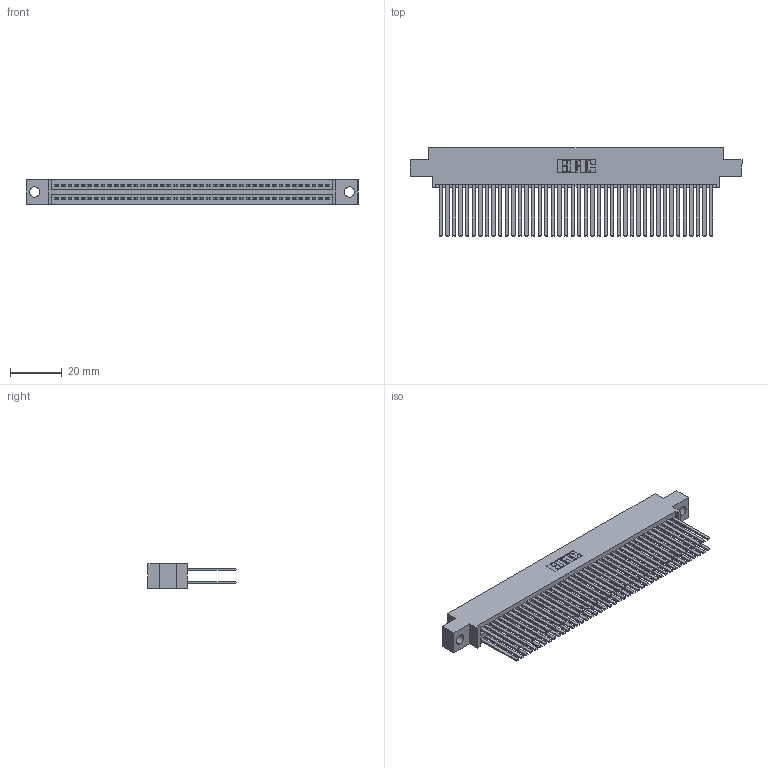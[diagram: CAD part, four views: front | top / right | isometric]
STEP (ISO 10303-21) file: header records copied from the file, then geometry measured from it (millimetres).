
FILE_DESCRIPTION (( 'STEP AP203' ), '1' );
FILE_NAME ('395-084-544-804.STEP', '2021-06-17T08:25:13', ( '' ), ( '' ), 'SwSTEP 2.0', 'SolidWorks 2020', '' );
FILE_SCHEMA (( 'CONFIG_CONTROL_DESIGN' ));
Length unit declared in the file: inch
Products named in the file (3): 345-292-001_345-293-144; 345 Part_0.170 Offset - 0.156 Dia-TI; 395-084-544-804
Assembly tree (85 placements, depth 2):
  395-084-544-804
    345 Part_0.170 Offset - 0.156 Dia-TI
    345-292-001_345-293-144  x84
Bounding box: 127.89 x 33.96 x 9.4 mm (x, y, z)
Volume: 13381.5 mm3; surface area: 23226.3 mm2
Topology: 85 solids, 85 shells, 3840 faces, 11393 edges, 7482 vertices
Faces by surface type: plane 2534, cylinder 1306
Entity records: 33321 total; most frequent: CARTESIAN_POINT 5590, ORIENTED_EDGE 5522, DIRECTION 4925, EDGE_CURVE 2761, VECTOR 2465, LINE 2465, VERTEX_POINT 1838, AXIS2_PLACEMENT_3D 1230
